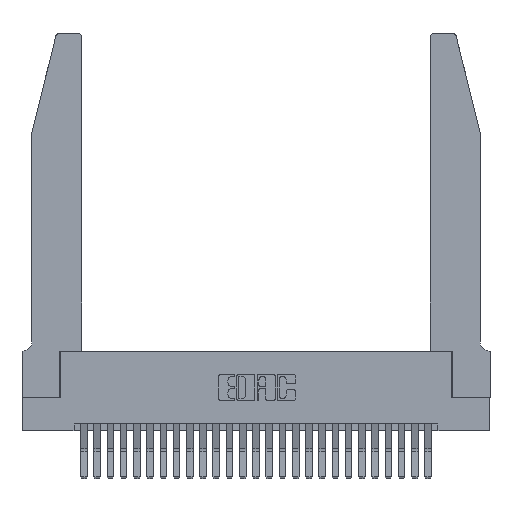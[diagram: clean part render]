
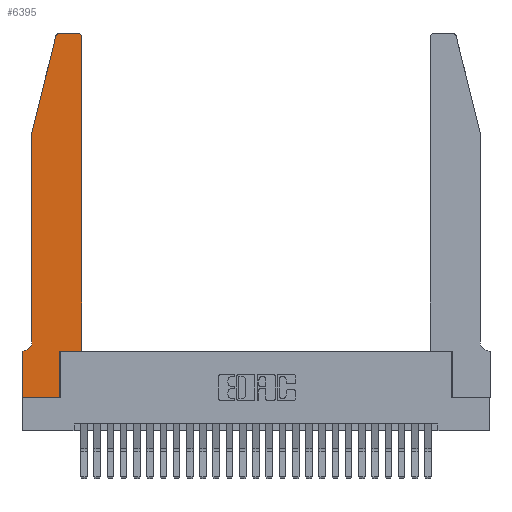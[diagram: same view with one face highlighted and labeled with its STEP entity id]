
A CAD part, top view. The second image highlights one B-rep face of the part: STEP entity #6395.
In plain terms, the highlighted planar face has unit normal (0, 0, 1).
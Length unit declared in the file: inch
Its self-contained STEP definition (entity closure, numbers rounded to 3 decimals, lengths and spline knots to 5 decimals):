
#19 = LINE ( 'NONE', #7922, #17573 ) ;
#243 = VECTOR ( 'NONE', #13610, 39.37008 ) ;
#823 = EDGE_CURVE ( 'NONE', #8872, #25315, #27500, .T. ) ;
#1039 = DIRECTION ( 'NONE',  ( -1., 0., 0. ) ) ;
#1232 = AXIS2_PLACEMENT_3D ( 'NONE', #26993, #14222, #1039 ) ;
#2168 = LINE ( 'NONE', #23642, #7368 ) ;
#2404 = CARTESIAN_POINT ( 'NONE',  ( 0.4205, 2.75, 0.37 ) ) ;
#3063 = VECTOR ( 'NONE', #15574, 39.37008 ) ;
#3828 = CARTESIAN_POINT ( 'NONE',  ( 0.25487, 2.72718, 0.37 ) ) ;
#4492 = EDGE_CURVE ( 'NONE', #18711, #20319, #10889, .T. ) ;
#4803 = CARTESIAN_POINT ( 'NONE',  ( 0.2865, 0., 0.37 ) ) ;
#5001 = AXIS2_PLACEMENT_3D ( 'NONE', #7336, #22458, #9529 ) ;
#5059 = ORIENTED_EDGE ( 'NONE', *, *, #25492, .T. ) ;
#5571 = CARTESIAN_POINT ( 'NONE',  ( 0., 0.35, 0.37 ) ) ;
#5920 = EDGE_CURVE ( 'NONE', #14548, #18079, #11884, .T. ) ;
#6164 = CARTESIAN_POINT ( 'NONE',  ( 0., 0.35, 0.37 ) ) ;
#6199 = CARTESIAN_POINT ( 'NONE',  ( 0.284, 2.75, 0.37 ) ) ;
#6395 = ADVANCED_FACE ( 'NONE', ( #18309 ), #19223, .T. ) ;
#6796 = DIRECTION ( 'NONE',  ( 0., 0., 1. ) ) ;
#6872 = LINE ( 'NONE', #11405, #243 ) ;
#7336 = CARTESIAN_POINT ( 'NONE',  ( 0.284, 2.72, 0.37 ) ) ;
#7368 = VECTOR ( 'NONE', #10761, 39.37008 ) ;
#7417 = CIRCLE ( 'NONE', #1232, 0.07 ) ;
#7922 = CARTESIAN_POINT ( 'NONE',  ( 0., 0., 0.37 ) ) ;
#8398 = DIRECTION ( 'NONE',  ( 0., 0., 1. ) ) ;
#8604 = AXIS2_PLACEMENT_3D ( 'NONE', #19815, #6796, #21963 ) ;
#8872 = VERTEX_POINT ( 'NONE', #10152 ) ;
#9529 = DIRECTION ( 'NONE',  ( 1., 0., 0. ) ) ;
#9650 = CARTESIAN_POINT ( 'NONE',  ( 0.4505, 0.35, 0.37 ) ) ;
#9726 = DIRECTION ( 'NONE',  ( -1., 0., 0. ) ) ;
#9772 = EDGE_CURVE ( 'NONE', #16655, #11549, #23639, .T. ) ;
#9806 = ORIENTED_EDGE ( 'NONE', *, *, #10004, .T. ) ;
#10004 = EDGE_CURVE ( 'NONE', #26102, #16655, #25004, .T. ) ;
#10152 = CARTESIAN_POINT ( 'NONE',  ( 0.0055, 0.35, 0.37 ) ) ;
#10736 = CARTESIAN_POINT ( 'NONE',  ( 0.2865, 0.35, 0.37 ) ) ;
#10761 = DIRECTION ( 'NONE',  ( 0., 1., 0. ) ) ;
#10860 = ORIENTED_EDGE ( 'NONE', *, *, #4492, .T. ) ;
#10889 = LINE ( 'NONE', #9650, #16012 ) ;
#11287 = CARTESIAN_POINT ( 'NONE',  ( 0.0755, 2., 0.37 ) ) ;
#11319 = EDGE_CURVE ( 'NONE', #24008, #8872, #7417, .T. ) ;
#11405 = CARTESIAN_POINT ( 'NONE',  ( 0.2605, 2.75, 0.37 ) ) ;
#11549 = VERTEX_POINT ( 'NONE', #11890 ) ;
#11879 = ORIENTED_EDGE ( 'NONE', *, *, #823, .T. ) ;
#11884 = CIRCLE ( 'NONE', #8604, 0.03 ) ;
#11890 = CARTESIAN_POINT ( 'NONE',  ( 0.0755, 2., 0.37 ) ) ;
#12117 = EDGE_LOOP ( 'NONE', ( #24952, #9806, #15628, #21329, #22647, #11879, #18995, #25963, #5059, #10860, #16649, #23645 ) ) ;
#12269 = EDGE_CURVE ( 'NONE', #25315, #22353, #19, .T. ) ;
#13610 = DIRECTION ( 'NONE',  ( -1., 0., 0. ) ) ;
#14222 = DIRECTION ( 'NONE',  ( 0., 0., -1. ) ) ;
#14548 = VERTEX_POINT ( 'NONE', #18433 ) ;
#14708 = LINE ( 'NONE', #11287, #3063 ) ;
#14910 = VERTEX_POINT ( 'NONE', #4803 ) ;
#15350 = CARTESIAN_POINT ( 'NONE',  ( 0.0755, 2., 0.37 ) ) ;
#15574 = DIRECTION ( 'NONE',  ( 0., -1., 0. ) ) ;
#15628 = ORIENTED_EDGE ( 'NONE', *, *, #9772, .T. ) ;
#15667 = VECTOR ( 'NONE', #25023, 39.37008 ) ;
#15977 = CARTESIAN_POINT ( 'NONE',  ( 0.0755, 0.35, 0.37 ) ) ;
#16012 = VECTOR ( 'NONE', #26815, 39.37008 ) ;
#16336 = LINE ( 'NONE', #18535, #15667 ) ;
#16649 = ORIENTED_EDGE ( 'NONE', *, *, #23171, .T. ) ;
#16655 = VERTEX_POINT ( 'NONE', #3828 ) ;
#17573 = VECTOR ( 'NONE', #23015, 39.37008 ) ;
#17689 = CARTESIAN_POINT ( 'NONE',  ( 0.2865, 0.35, 0.37 ) ) ;
#18017 = VECTOR ( 'NONE', #19698, 39.37008 ) ;
#18079 = VERTEX_POINT ( 'NONE', #2404 ) ;
#18136 = CARTESIAN_POINT ( 'NONE',  ( 0.0755, 0.42, 0.37 ) ) ;
#18309 = FACE_OUTER_BOUND ( 'NONE', #12117, .T. ) ;
#18433 = CARTESIAN_POINT ( 'NONE',  ( 0.4505, 2.72, 0.37 ) ) ;
#18535 = CARTESIAN_POINT ( 'NONE',  ( 0., 0., 0.37 ) ) ;
#18711 = VERTEX_POINT ( 'NONE', #17689 ) ;
#18787 = VECTOR ( 'NONE', #23613, 39.37008 ) ;
#18995 = ORIENTED_EDGE ( 'NONE', *, *, #12269, .T. ) ;
#19223 = PLANE ( 'NONE',  #25361 ) ;
#19404 = EDGE_CURVE ( 'NONE', #11549, #24008, #14708, .T. ) ;
#19482 = LINE ( 'NONE', #10736, #18787 ) ;
#19698 = DIRECTION ( 'NONE',  ( -0.239, -0.971, 0. ) ) ;
#19815 = CARTESIAN_POINT ( 'NONE',  ( 0.4205, 2.72, 0.37 ) ) ;
#20319 = VERTEX_POINT ( 'NONE', #27720 ) ;
#21329 = ORIENTED_EDGE ( 'NONE', *, *, #19404, .T. ) ;
#21934 = VECTOR ( 'NONE', #9726, 39.37008 ) ;
#21963 = DIRECTION ( 'NONE',  ( 1., 0., 0. ) ) ;
#22353 = VERTEX_POINT ( 'NONE', #24437 ) ;
#22458 = DIRECTION ( 'NONE',  ( 0., 0., 1. ) ) ;
#22647 = ORIENTED_EDGE ( 'NONE', *, *, #11319, .T. ) ;
#23015 = DIRECTION ( 'NONE',  ( 0., -1., 0. ) ) ;
#23171 = EDGE_CURVE ( 'NONE', #20319, #14548, #2168, .T. ) ;
#23474 = DIRECTION ( 'NONE',  ( 1., 0., 0. ) ) ;
#23613 = DIRECTION ( 'NONE',  ( 0., 1., 0. ) ) ;
#23639 = LINE ( 'NONE', #15350, #18017 ) ;
#23642 = CARTESIAN_POINT ( 'NONE',  ( 0.4505, 0.35, 0.37 ) ) ;
#23645 = ORIENTED_EDGE ( 'NONE', *, *, #5920, .T. ) ;
#24008 = VERTEX_POINT ( 'NONE', #18136 ) ;
#24437 = CARTESIAN_POINT ( 'NONE',  ( 0., 0., 0.37 ) ) ;
#24952 = ORIENTED_EDGE ( 'NONE', *, *, #25719, .T. ) ;
#25004 = CIRCLE ( 'NONE', #5001, 0.03 ) ;
#25023 = DIRECTION ( 'NONE',  ( 1., 0., 0. ) ) ;
#25315 = VERTEX_POINT ( 'NONE', #5571 ) ;
#25361 = AXIS2_PLACEMENT_3D ( 'NONE', #6164, #8398, #23474 ) ;
#25492 = EDGE_CURVE ( 'NONE', #14910, #18711, #19482, .T. ) ;
#25719 = EDGE_CURVE ( 'NONE', #18079, #26102, #6872, .T. ) ;
#25963 = ORIENTED_EDGE ( 'NONE', *, *, #27122, .T. ) ;
#26102 = VERTEX_POINT ( 'NONE', #6199 ) ;
#26815 = DIRECTION ( 'NONE',  ( 1., 0., 0. ) ) ;
#26993 = CARTESIAN_POINT ( 'NONE',  ( 0.0055, 0.42, 0.37 ) ) ;
#27122 = EDGE_CURVE ( 'NONE', #22353, #14910, #16336, .T. ) ;
#27500 = LINE ( 'NONE', #15977, #21934 ) ;
#27720 = CARTESIAN_POINT ( 'NONE',  ( 0.4505, 0.35, 0.37 ) ) ;
